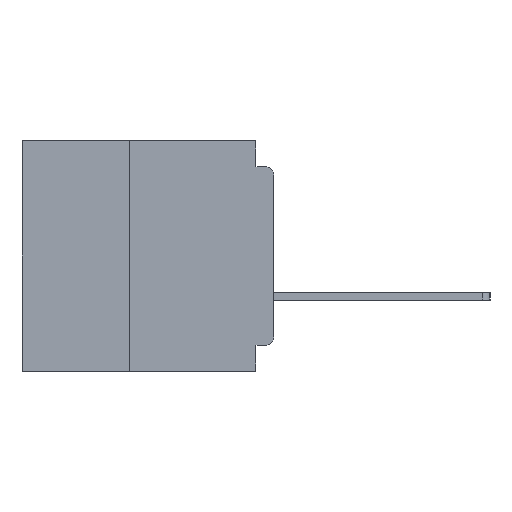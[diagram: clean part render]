
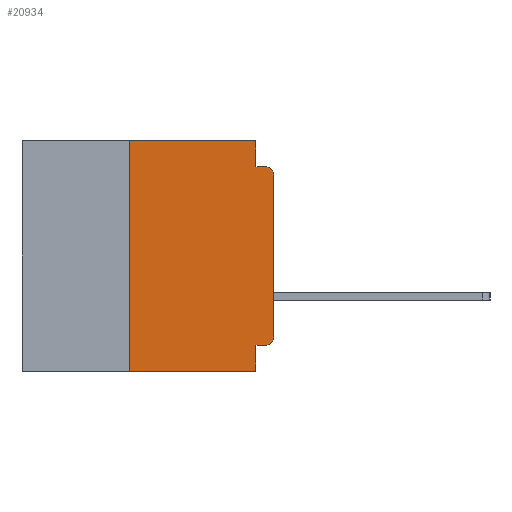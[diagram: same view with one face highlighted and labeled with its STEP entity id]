
A CAD part, left-side view. The second image highlights one B-rep face of the part: STEP entity #20934.
In plain terms, the highlighted planar face has unit normal (-1, 0, 0).
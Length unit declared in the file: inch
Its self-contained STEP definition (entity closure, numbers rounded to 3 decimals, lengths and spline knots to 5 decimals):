
#113 = EDGE_CURVE ( 'NONE', #15126, #13097, #9405, .T. ) ;
#193 = DIRECTION ( 'NONE',  ( 0., 0., 1. ) ) ;
#681 = CARTESIAN_POINT ( 'NONE',  ( 0., 0.437, -0.4 ) ) ;
#923 = DIRECTION ( 'NONE',  ( 0., -1., 0. ) ) ;
#2276 = CARTESIAN_POINT ( 'NONE',  ( 0., 0.031, -0.045 ) ) ;
#2974 = DIRECTION ( 'NONE',  ( 0., 0., 1. ) ) ;
#4218 = VERTEX_POINT ( 'NONE', #8627 ) ;
#5010 = EDGE_LOOP ( 'NONE', ( #43212, #15169, #33636, #36306, #51310, #37478, #45222, #35737, #25200, #27001 ) ) ;
#5454 = VERTEX_POINT ( 'NONE', #16822 ) ;
#6028 = CARTESIAN_POINT ( 'NONE',  ( 0., 0., -0.355 ) ) ;
#6724 = VECTOR ( 'NONE', #923, 39.37008 ) ;
#6773 = CARTESIAN_POINT ( 'NONE',  ( 0., 0.015, -0.06 ) ) ;
#6776 = EDGE_CURVE ( 'NONE', #39784, #14653, #55177, .T. ) ;
#6804 = CARTESIAN_POINT ( 'NONE',  ( 0., 0.25, -0.4 ) ) ;
#7629 = VECTOR ( 'NONE', #17526, 39.37008 ) ;
#7747 = VECTOR ( 'NONE', #2974, 39.37008 ) ;
#7979 = PLANE ( 'NONE',  #40275 ) ;
#8147 = DIRECTION ( 'NONE',  ( 1., 0., 0. ) ) ;
#8426 = AXIS2_PLACEMENT_3D ( 'NONE', #38832, #12916, #43185 ) ;
#8627 = CARTESIAN_POINT ( 'NONE',  ( 0., 0., -0.34 ) ) ;
#9101 = VECTOR ( 'NONE', #21441, 39.37008 ) ;
#9405 = LINE ( 'NONE', #681, #6724 ) ;
#10373 = DIRECTION ( 'NONE',  ( 0., 1., 0. ) ) ;
#10392 = CARTESIAN_POINT ( 'NONE',  ( 0., 0.031, -0.355 ) ) ;
#11115 = DIRECTION ( 'NONE',  ( 0., 0., -1. ) ) ;
#11474 = LINE ( 'NONE', #42129, #33150 ) ;
#12916 = DIRECTION ( 'NONE',  ( -1., 0., 0. ) ) ;
#13097 = VERTEX_POINT ( 'NONE', #39055 ) ;
#14653 = VERTEX_POINT ( 'NONE', #16479 ) ;
#15126 = VERTEX_POINT ( 'NONE', #6804 ) ;
#15169 = ORIENTED_EDGE ( 'NONE', *, *, #32478, .T. ) ;
#15286 = LINE ( 'NONE', #21620, #41045 ) ;
#16479 = CARTESIAN_POINT ( 'NONE',  ( 0., 0.031, 0. ) ) ;
#16822 = CARTESIAN_POINT ( 'NONE',  ( 0., 0.015, -0.355 ) ) ;
#17074 = EDGE_CURVE ( 'NONE', #15126, #39784, #29421, .T. ) ;
#17526 = DIRECTION ( 'NONE',  ( 0., 0., -1. ) ) ;
#19127 = CIRCLE ( 'NONE', #8426, 0.015 ) ;
#20541 = DIRECTION ( 'NONE',  ( 0., -1., 0. ) ) ;
#20934 = ADVANCED_FACE ( 'NONE', ( #22216 ), #7979, .F. ) ;
#21441 = DIRECTION ( 'NONE',  ( 0., -1., 0. ) ) ;
#21620 = CARTESIAN_POINT ( 'NONE',  ( 0., 0., 0. ) ) ;
#22216 = FACE_OUTER_BOUND ( 'NONE', #5010, .T. ) ;
#22245 = CARTESIAN_POINT ( 'NONE',  ( 0., 0.25, 0. ) ) ;
#22414 = VERTEX_POINT ( 'NONE', #52632 ) ;
#22562 = DIRECTION ( 'NONE',  ( 0., 0., -1. ) ) ;
#24116 = AXIS2_PLACEMENT_3D ( 'NONE', #6773, #37036, #11115 ) ;
#25200 = ORIENTED_EDGE ( 'NONE', *, *, #30410, .F. ) ;
#25984 = VECTOR ( 'NONE', #10373, 39.37008 ) ;
#26094 = CARTESIAN_POINT ( 'NONE',  ( 0., 0.031, 0. ) ) ;
#27001 = ORIENTED_EDGE ( 'NONE', *, *, #49635, .T. ) ;
#29421 = LINE ( 'NONE', #46157, #7747 ) ;
#29698 = CARTESIAN_POINT ( 'NONE',  ( 0., 0., -0.06 ) ) ;
#29709 = EDGE_CURVE ( 'NONE', #34134, #13097, #51073, .T. ) ;
#29739 = CARTESIAN_POINT ( 'NONE',  ( 0., 0.437, 0. ) ) ;
#29857 = VERTEX_POINT ( 'NONE', #2276 ) ;
#30186 = CARTESIAN_POINT ( 'NONE',  ( 0., 0.437, 0. ) ) ;
#30410 = EDGE_CURVE ( 'NONE', #5454, #34134, #31405, .T. ) ;
#31405 = LINE ( 'NONE', #6028, #25984 ) ;
#32478 = EDGE_CURVE ( 'NONE', #41256, #22414, #51418, .T. ) ;
#32582 = EDGE_CURVE ( 'NONE', #29857, #22414, #11474, .T. ) ;
#33150 = VECTOR ( 'NONE', #20541, 39.37008 ) ;
#33636 = ORIENTED_EDGE ( 'NONE', *, *, #32582, .F. ) ;
#34134 = VERTEX_POINT ( 'NONE', #10392 ) ;
#35737 = ORIENTED_EDGE ( 'NONE', *, *, #29709, .F. ) ;
#36275 = EDGE_CURVE ( 'NONE', #14653, #29857, #53657, .T. ) ;
#36306 = ORIENTED_EDGE ( 'NONE', *, *, #36275, .F. ) ;
#37036 = DIRECTION ( 'NONE',  ( -1., 0., 0. ) ) ;
#37478 = ORIENTED_EDGE ( 'NONE', *, *, #17074, .F. ) ;
#38426 = DIRECTION ( 'NONE',  ( 0., 0., -1. ) ) ;
#38832 = CARTESIAN_POINT ( 'NONE',  ( 0., 0.015, -0.34 ) ) ;
#39055 = CARTESIAN_POINT ( 'NONE',  ( 0., 0.031, -0.4 ) ) ;
#39573 = VECTOR ( 'NONE', #22562, 39.37008 ) ;
#39784 = VERTEX_POINT ( 'NONE', #22245 ) ;
#40275 = AXIS2_PLACEMENT_3D ( 'NONE', #29739, #8147, #38426 ) ;
#41045 = VECTOR ( 'NONE', #193, 39.37008 ) ;
#41256 = VERTEX_POINT ( 'NONE', #29698 ) ;
#42001 = EDGE_CURVE ( 'NONE', #4218, #41256, #15286, .T. ) ;
#42129 = CARTESIAN_POINT ( 'NONE',  ( 0., 0., -0.045 ) ) ;
#43185 = DIRECTION ( 'NONE',  ( 0., 0., -1. ) ) ;
#43212 = ORIENTED_EDGE ( 'NONE', *, *, #42001, .T. ) ;
#45222 = ORIENTED_EDGE ( 'NONE', *, *, #113, .T. ) ;
#46157 = CARTESIAN_POINT ( 'NONE',  ( 0., 0.25, -0.4 ) ) ;
#49635 = EDGE_CURVE ( 'NONE', #5454, #4218, #19127, .T. ) ;
#51073 = LINE ( 'NONE', #52829, #39573 ) ;
#51310 = ORIENTED_EDGE ( 'NONE', *, *, #6776, .F. ) ;
#51418 = CIRCLE ( 'NONE', #24116, 0.015 ) ;
#52632 = CARTESIAN_POINT ( 'NONE',  ( 0., 0.015, -0.045 ) ) ;
#52829 = CARTESIAN_POINT ( 'NONE',  ( 0., 0.031, -0.4 ) ) ;
#53657 = LINE ( 'NONE', #26094, #7629 ) ;
#55177 = LINE ( 'NONE', #30186, #9101 ) ;
